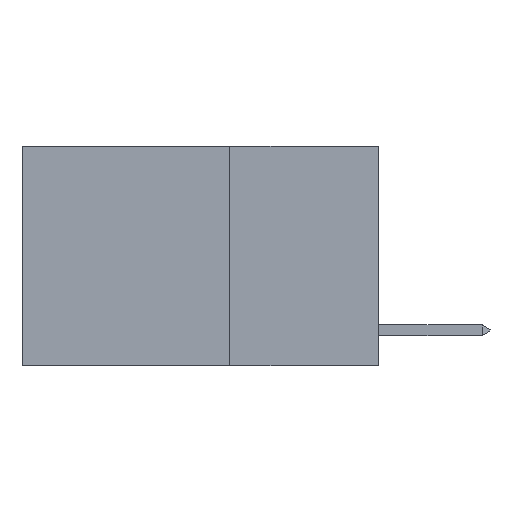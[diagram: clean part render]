
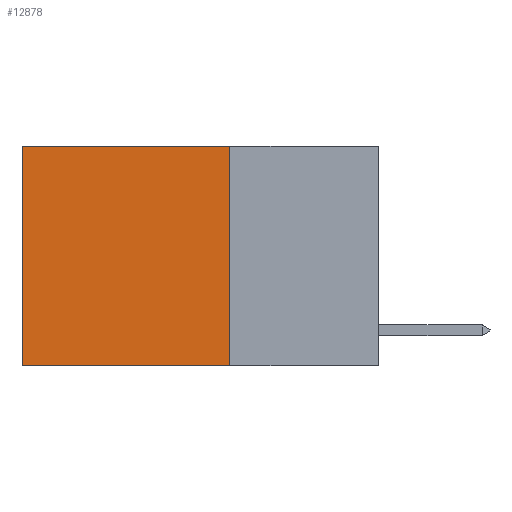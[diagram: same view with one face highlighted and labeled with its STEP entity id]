
A CAD part, left-side view. The second image highlights one B-rep face of the part: STEP entity #12878.
In plain terms, the highlighted planar face has unit normal (-1, 0, 0).
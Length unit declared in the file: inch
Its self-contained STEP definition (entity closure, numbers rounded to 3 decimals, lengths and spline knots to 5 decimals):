
#230 = CARTESIAN_POINT ( 'NONE',  ( 0.2625, 0.25, 0. ) ) ;
#696 = CARTESIAN_POINT ( 'NONE',  ( 0.2625, 0.25, -0.37 ) ) ;
#1153 = VERTEX_POINT ( 'NONE', #696 ) ;
#1225 = LINE ( 'NONE', #4842, #14379 ) ;
#1588 = LINE ( 'NONE', #14340, #11761 ) ;
#1991 = EDGE_LOOP ( 'NONE', ( #6533, #14934, #2909, #2289 ) ) ;
#2289 = ORIENTED_EDGE ( 'NONE', *, *, #7096, .T. ) ;
#2660 = DIRECTION ( 'NONE',  ( 0., 0., -1. ) ) ;
#2909 = ORIENTED_EDGE ( 'NONE', *, *, #3893, .F. ) ;
#2924 = DIRECTION ( 'NONE',  ( 0., 0., -1. ) ) ;
#3032 = CARTESIAN_POINT ( 'NONE',  ( 0.2625, 0.25, 0. ) ) ;
#3893 = EDGE_CURVE ( 'NONE', #14609, #1153, #5936, .T. ) ;
#4218 = CARTESIAN_POINT ( 'NONE',  ( 0.2625, 0.25, 0. ) ) ;
#4475 = EDGE_CURVE ( 'NONE', #1153, #5283, #1588, .T. ) ;
#4842 = CARTESIAN_POINT ( 'NONE',  ( 0.2625, 0.25, 0. ) ) ;
#5283 = VERTEX_POINT ( 'NONE', #13937 ) ;
#5298 = EDGE_CURVE ( 'NONE', #14419, #5283, #5883, .T. ) ;
#5775 = FACE_OUTER_BOUND ( 'NONE', #1991, .T. ) ;
#5883 = LINE ( 'NONE', #13438, #15828 ) ;
#5936 = LINE ( 'NONE', #3032, #15491 ) ;
#6533 = ORIENTED_EDGE ( 'NONE', *, *, #5298, .T. ) ;
#7096 = EDGE_CURVE ( 'NONE', #14609, #14419, #1225, .T. ) ;
#7161 = AXIS2_PLACEMENT_3D ( 'NONE', #230, #10543, #2924 ) ;
#9262 = PLANE ( 'NONE',  #7161 ) ;
#10543 = DIRECTION ( 'NONE',  ( 1., 0., 0. ) ) ;
#11761 = VECTOR ( 'NONE', #14363, 39.37008 ) ;
#12641 = CARTESIAN_POINT ( 'NONE',  ( 0.2625, 0.6, 0. ) ) ;
#12878 = ADVANCED_FACE ( 'NONE', ( #5775 ), #9262, .F. ) ;
#13232 = DIRECTION ( 'NONE',  ( 0., 0., -1. ) ) ;
#13438 = CARTESIAN_POINT ( 'NONE',  ( 0.2625, 0.6, 0. ) ) ;
#13937 = CARTESIAN_POINT ( 'NONE',  ( 0.2625, 0.6, -0.37 ) ) ;
#14340 = CARTESIAN_POINT ( 'NONE',  ( 0.2625, 0.25, -0.37 ) ) ;
#14363 = DIRECTION ( 'NONE',  ( 0., 1., 0. ) ) ;
#14379 = VECTOR ( 'NONE', #14887, 39.37008 ) ;
#14419 = VERTEX_POINT ( 'NONE', #12641 ) ;
#14609 = VERTEX_POINT ( 'NONE', #4218 ) ;
#14887 = DIRECTION ( 'NONE',  ( 0., 1., 0. ) ) ;
#14934 = ORIENTED_EDGE ( 'NONE', *, *, #4475, .F. ) ;
#15491 = VECTOR ( 'NONE', #2660, 39.37008 ) ;
#15828 = VECTOR ( 'NONE', #13232, 39.37008 ) ;
